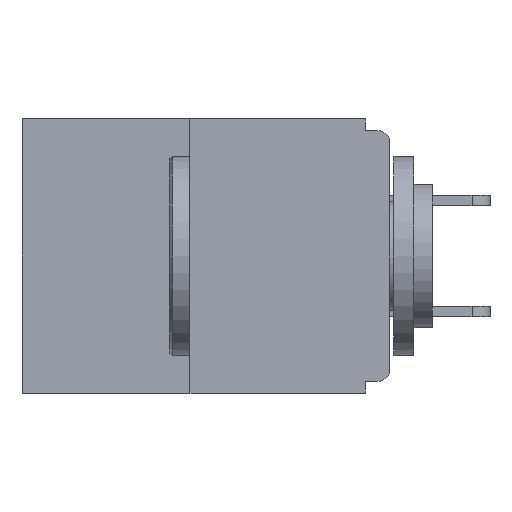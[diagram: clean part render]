
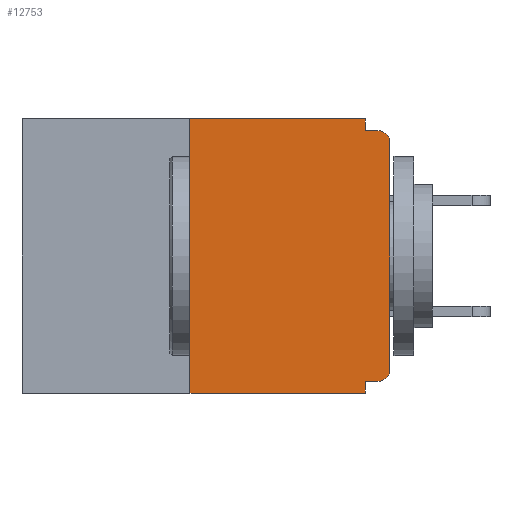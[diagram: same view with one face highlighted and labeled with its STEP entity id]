
A CAD part, left-side view. The second image highlights one B-rep face of the part: STEP entity #12753.
In plain terms, the highlighted planar face has unit normal (-1, 0, 0).
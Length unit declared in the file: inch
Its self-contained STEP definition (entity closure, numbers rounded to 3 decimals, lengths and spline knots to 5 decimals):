
#144 = CIRCLE ( 'NONE', #3081, 0.015 ) ;
#340 = VECTOR ( 'NONE', #13103, 39.37008 ) ;
#570 = VECTOR ( 'NONE', #7650, 39.37008 ) ;
#669 = VECTOR ( 'NONE', #5796, 39.37008 ) ;
#790 = VERTEX_POINT ( 'NONE', #5450 ) ;
#837 = ORIENTED_EDGE ( 'NONE', *, *, #6796, .F. ) ;
#1519 = VECTOR ( 'NONE', #2794, 39.37008 ) ;
#1636 = VERTEX_POINT ( 'NONE', #10431 ) ;
#1846 = CARTESIAN_POINT ( 'NONE',  ( 0., 0., -0.015 ) ) ;
#2069 = DIRECTION ( 'NONE',  ( 1., 0., 0. ) ) ;
#2231 = LINE ( 'NONE', #3330, #570 ) ;
#2794 = DIRECTION ( 'NONE',  ( 0., 1., 0. ) ) ;
#2835 = LINE ( 'NONE', #3955, #6652 ) ;
#2867 = PLANE ( 'NONE',  #6947 ) ;
#2879 = CARTESIAN_POINT ( 'NONE',  ( 0., 0., -0.03 ) ) ;
#2972 = EDGE_CURVE ( 'NONE', #790, #9461, #10349, .T. ) ;
#3081 = AXIS2_PLACEMENT_3D ( 'NONE', #12822, #6439, #5353 ) ;
#3258 = LINE ( 'NONE', #1846, #10263 ) ;
#3330 = CARTESIAN_POINT ( 'NONE',  ( 0., 0.46, -0.343 ) ) ;
#3502 = LINE ( 'NONE', #3541, #340 ) ;
#3541 = CARTESIAN_POINT ( 'NONE',  ( 0., 0.46, 0. ) ) ;
#3955 = CARTESIAN_POINT ( 'NONE',  ( 0., 0.031, 0. ) ) ;
#3973 = EDGE_CURVE ( 'NONE', #8142, #12536, #8243, .T. ) ;
#4003 = DIRECTION ( 'NONE',  ( -1., 0., 0. ) ) ;
#4097 = VERTEX_POINT ( 'NONE', #10438 ) ;
#4173 = LINE ( 'NONE', #11068, #669 ) ;
#4797 = EDGE_CURVE ( 'NONE', #4097, #7829, #2231, .T. ) ;
#4993 = CARTESIAN_POINT ( 'NONE',  ( 0., 0., -0.328 ) ) ;
#5086 = ORIENTED_EDGE ( 'NONE', *, *, #3973, .T. ) ;
#5149 = ORIENTED_EDGE ( 'NONE', *, *, #8686, .F. ) ;
#5256 = VERTEX_POINT ( 'NONE', #7617 ) ;
#5353 = DIRECTION ( 'NONE',  ( 0., 0., -1. ) ) ;
#5450 = CARTESIAN_POINT ( 'NONE',  ( 0., 0.015, -0.328 ) ) ;
#5796 = DIRECTION ( 'NONE',  ( 0., 0., -1. ) ) ;
#6019 = VERTEX_POINT ( 'NONE', #12106 ) ;
#6037 = DIRECTION ( 'NONE',  ( 0., -1., 0. ) ) ;
#6117 = LINE ( 'NONE', #9421, #6618 ) ;
#6120 = CARTESIAN_POINT ( 'NONE',  ( 0., 0.015, -0.03 ) ) ;
#6126 = LINE ( 'NONE', #8388, #7281 ) ;
#6267 = ORIENTED_EDGE ( 'NONE', *, *, #12479, .F. ) ;
#6439 = DIRECTION ( 'NONE',  ( -1., 0., 0. ) ) ;
#6618 = VECTOR ( 'NONE', #11539, 39.37008 ) ;
#6652 = VECTOR ( 'NONE', #9189, 39.37008 ) ;
#6796 = EDGE_CURVE ( 'NONE', #1636, #6019, #3502, .T. ) ;
#6856 = EDGE_CURVE ( 'NONE', #6019, #5256, #2835, .T. ) ;
#6947 = AXIS2_PLACEMENT_3D ( 'NONE', #9523, #2069, #12583 ) ;
#6992 = VERTEX_POINT ( 'NONE', #13681 ) ;
#7062 = AXIS2_PLACEMENT_3D ( 'NONE', #6120, #4003, #8258 ) ;
#7166 = EDGE_CURVE ( 'NONE', #9461, #7829, #4173, .T. ) ;
#7281 = VECTOR ( 'NONE', #9512, 39.37008 ) ;
#7617 = CARTESIAN_POINT ( 'NONE',  ( 0., 0.031, -0.015 ) ) ;
#7650 = DIRECTION ( 'NONE',  ( 0., -1., 0. ) ) ;
#7741 = EDGE_CURVE ( 'NONE', #6992, #8142, #6126, .T. ) ;
#7829 = VERTEX_POINT ( 'NONE', #10915 ) ;
#8142 = VERTEX_POINT ( 'NONE', #2879 ) ;
#8243 = CIRCLE ( 'NONE', #7062, 0.015 ) ;
#8258 = DIRECTION ( 'NONE',  ( 0., 0., -1. ) ) ;
#8388 = CARTESIAN_POINT ( 'NONE',  ( 0., 0., 0. ) ) ;
#8439 = CARTESIAN_POINT ( 'NONE',  ( 0., 0.031, -0.328 ) ) ;
#8572 = EDGE_CURVE ( 'NONE', #790, #6992, #144, .T. ) ;
#8686 = EDGE_CURVE ( 'NONE', #4097, #1636, #6117, .T. ) ;
#9189 = DIRECTION ( 'NONE',  ( 0., 0., -1. ) ) ;
#9282 = CARTESIAN_POINT ( 'NONE',  ( 0., 0.015, -0.015 ) ) ;
#9320 = ORIENTED_EDGE ( 'NONE', *, *, #7166, .F. ) ;
#9421 = CARTESIAN_POINT ( 'NONE',  ( 0., 0.25, 0. ) ) ;
#9461 = VERTEX_POINT ( 'NONE', #8439 ) ;
#9512 = DIRECTION ( 'NONE',  ( 0., 0., 1. ) ) ;
#9523 = CARTESIAN_POINT ( 'NONE',  ( 0., 0.46, 0. ) ) ;
#10263 = VECTOR ( 'NONE', #6037, 39.37008 ) ;
#10349 = LINE ( 'NONE', #4993, #1519 ) ;
#10428 = ORIENTED_EDGE ( 'NONE', *, *, #6856, .F. ) ;
#10431 = CARTESIAN_POINT ( 'NONE',  ( 0., 0.25, 0. ) ) ;
#10438 = CARTESIAN_POINT ( 'NONE',  ( 0., 0.25, -0.343 ) ) ;
#10791 = ORIENTED_EDGE ( 'NONE', *, *, #4797, .T. ) ;
#10915 = CARTESIAN_POINT ( 'NONE',  ( 0., 0.031, -0.343 ) ) ;
#11068 = CARTESIAN_POINT ( 'NONE',  ( 0., 0.031, -0.343 ) ) ;
#11539 = DIRECTION ( 'NONE',  ( 0., 0., 1. ) ) ;
#11570 = ORIENTED_EDGE ( 'NONE', *, *, #8572, .T. ) ;
#12106 = CARTESIAN_POINT ( 'NONE',  ( 0., 0.031, 0. ) ) ;
#12479 = EDGE_CURVE ( 'NONE', #5256, #12536, #3258, .T. ) ;
#12536 = VERTEX_POINT ( 'NONE', #9282 ) ;
#12583 = DIRECTION ( 'NONE',  ( 0., 0., -1. ) ) ;
#12632 = ORIENTED_EDGE ( 'NONE', *, *, #2972, .F. ) ;
#12753 = ADVANCED_FACE ( 'NONE', ( #13722 ), #2867, .F. ) ;
#12769 = ORIENTED_EDGE ( 'NONE', *, *, #7741, .T. ) ;
#12822 = CARTESIAN_POINT ( 'NONE',  ( 0., 0.015, -0.313 ) ) ;
#13103 = DIRECTION ( 'NONE',  ( 0., -1., 0. ) ) ;
#13293 = EDGE_LOOP ( 'NONE', ( #837, #5149, #10791, #9320, #12632, #11570, #12769, #5086, #6267, #10428 ) ) ;
#13681 = CARTESIAN_POINT ( 'NONE',  ( 0., 0., -0.313 ) ) ;
#13722 = FACE_OUTER_BOUND ( 'NONE', #13293, .T. ) ;
